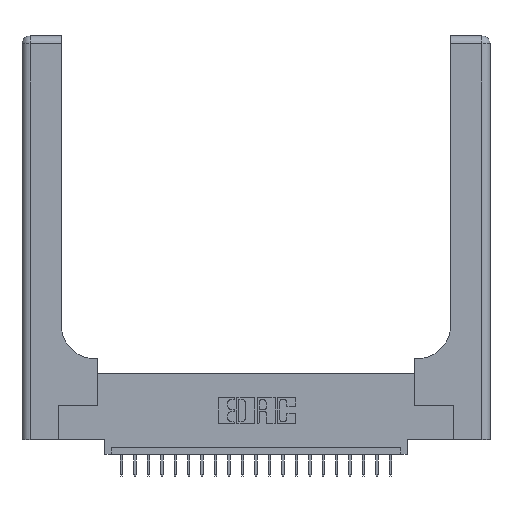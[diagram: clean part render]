
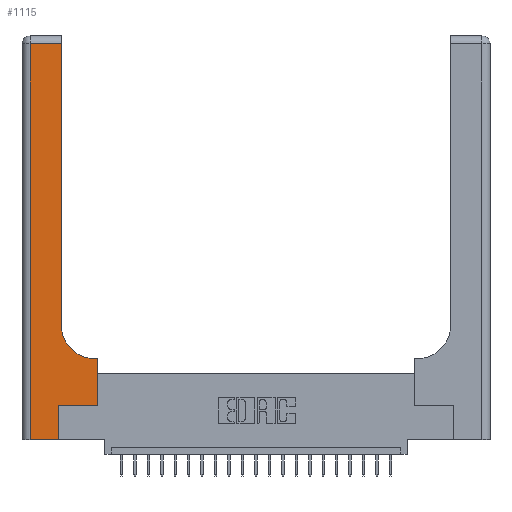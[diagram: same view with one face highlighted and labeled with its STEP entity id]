
A CAD part, top view. The second image highlights one B-rep face of the part: STEP entity #1115.
In plain terms, the highlighted planar face has unit normal (0, 0, 1).
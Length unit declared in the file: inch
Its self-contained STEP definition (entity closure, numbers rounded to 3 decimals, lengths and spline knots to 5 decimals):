
#96 = ORIENTED_EDGE ( 'NONE', *, *, #11299, .T. ) ;
#660 = VECTOR ( 'NONE', #7168, 39.37008 ) ;
#1115 = ADVANCED_FACE ( 'NONE', ( #14633 ), #4373, .F. ) ;
#1255 = VERTEX_POINT ( 'NONE', #6932 ) ;
#2038 = DIRECTION ( 'NONE',  ( 0., 1., 0. ) ) ;
#2277 = ORIENTED_EDGE ( 'NONE', *, *, #12733, .T. ) ;
#2320 = VECTOR ( 'NONE', #6712, 39.37008 ) ;
#2833 = DIRECTION ( 'NONE',  ( 1., 0., 0. ) ) ;
#3417 = ORIENTED_EDGE ( 'NONE', *, *, #20198, .T. ) ;
#3711 = DIRECTION ( 'NONE',  ( -1., 0., 0. ) ) ;
#3892 = ORIENTED_EDGE ( 'NONE', *, *, #22491, .T. ) ;
#4273 = EDGE_CURVE ( 'NONE', #1255, #19383, #12418, .T. ) ;
#4373 = PLANE ( 'NONE',  #24038 ) ;
#5080 = VECTOR ( 'NONE', #5881, 39.37008 ) ;
#5132 = EDGE_LOOP ( 'NONE', ( #2277, #96, #16296, #3892, #3417, #22652, #8991, #7483, #16198 ) ) ;
#5324 = LINE ( 'NONE', #10948, #6477 ) ;
#5587 = CARTESIAN_POINT ( 'NONE',  ( 0.2915, 0.85, 0.37 ) ) ;
#5657 = LINE ( 'NONE', #8108, #19506 ) ;
#5779 = AXIS2_PLACEMENT_3D ( 'NONE', #7704, #14783, #20620 ) ;
#5881 = DIRECTION ( 'NONE',  ( -1., 0., 0. ) ) ;
#6238 = CARTESIAN_POINT ( 'NONE',  ( 0., 3., 0.37 ) ) ;
#6273 = LINE ( 'NONE', #6801, #11749 ) ;
#6477 = VECTOR ( 'NONE', #2038, 39.37008 ) ;
#6712 = DIRECTION ( 'NONE',  ( 0., 1., 0. ) ) ;
#6801 = CARTESIAN_POINT ( 'NONE',  ( 0.269, 0., 0.37 ) ) ;
#6928 = CARTESIAN_POINT ( 'NONE',  ( 0.06, 2.94, 0.37 ) ) ;
#6932 = CARTESIAN_POINT ( 'NONE',  ( 0.5585, 0.25, 0.37 ) ) ;
#7168 = DIRECTION ( 'NONE',  ( 0., -1., 0. ) ) ;
#7483 = ORIENTED_EDGE ( 'NONE', *, *, #13497, .T. ) ;
#7704 = CARTESIAN_POINT ( 'NONE',  ( 0.5415, 0.85, 0.37 ) ) ;
#8108 = CARTESIAN_POINT ( 'NONE',  ( 0.269, 0.25, 0.37 ) ) ;
#8991 = ORIENTED_EDGE ( 'NONE', *, *, #4273, .T. ) ;
#10378 = VECTOR ( 'NONE', #14748, 39.37008 ) ;
#10526 = VERTEX_POINT ( 'NONE', #23783 ) ;
#10531 = VERTEX_POINT ( 'NONE', #14537 ) ;
#10604 = VERTEX_POINT ( 'NONE', #5587 ) ;
#10948 = CARTESIAN_POINT ( 'NONE',  ( 0.2915, 3., 0.37 ) ) ;
#11299 = EDGE_CURVE ( 'NONE', #10531, #23499, #14876, .T. ) ;
#11749 = VECTOR ( 'NONE', #21236, 39.37008 ) ;
#11845 = EDGE_CURVE ( 'NONE', #16604, #1255, #5657, .T. ) ;
#12418 = LINE ( 'NONE', #15806, #2320 ) ;
#12733 = EDGE_CURVE ( 'NONE', #10604, #10531, #5324, .T. ) ;
#12769 = VECTOR ( 'NONE', #3711, 39.37008 ) ;
#13497 = EDGE_CURVE ( 'NONE', #19383, #17892, #17670, .T. ) ;
#13524 = CARTESIAN_POINT ( 'NONE',  ( 0., 2.94, 0.37 ) ) ;
#13727 = DIRECTION ( 'NONE',  ( -1., 0., 0. ) ) ;
#13893 = EDGE_CURVE ( 'NONE', #17892, #10604, #22330, .T. ) ;
#14537 = CARTESIAN_POINT ( 'NONE',  ( 0.2915, 2.94, 0.37 ) ) ;
#14633 = FACE_OUTER_BOUND ( 'NONE', #5132, .T. ) ;
#14748 = DIRECTION ( 'NONE',  ( 1., 0., 0. ) ) ;
#14783 = DIRECTION ( 'NONE',  ( 0., 0., -1. ) ) ;
#14806 = CARTESIAN_POINT ( 'NONE',  ( 0.5585, 0.6, 0.37 ) ) ;
#14876 = LINE ( 'NONE', #13524, #5080 ) ;
#15123 = CARTESIAN_POINT ( 'NONE',  ( 0.269, 0.25, 0.37 ) ) ;
#15615 = EDGE_CURVE ( 'NONE', #23499, #16843, #17150, .T. ) ;
#15806 = CARTESIAN_POINT ( 'NONE',  ( 0.5585, 0.25, 0.37 ) ) ;
#16198 = ORIENTED_EDGE ( 'NONE', *, *, #13893, .T. ) ;
#16296 = ORIENTED_EDGE ( 'NONE', *, *, #15615, .T. ) ;
#16604 = VERTEX_POINT ( 'NONE', #15123 ) ;
#16655 = CARTESIAN_POINT ( 'NONE',  ( 0.06, 3., 0.37 ) ) ;
#16843 = VERTEX_POINT ( 'NONE', #21489 ) ;
#17150 = LINE ( 'NONE', #16655, #660 ) ;
#17456 = CARTESIAN_POINT ( 'NONE',  ( 0.5415, 0.6, 0.37 ) ) ;
#17670 = LINE ( 'NONE', #22539, #12769 ) ;
#17892 = VERTEX_POINT ( 'NONE', #17456 ) ;
#19132 = DIRECTION ( 'NONE',  ( 0., 0., -1. ) ) ;
#19383 = VERTEX_POINT ( 'NONE', #14806 ) ;
#19506 = VECTOR ( 'NONE', #2833, 39.37008 ) ;
#20198 = EDGE_CURVE ( 'NONE', #10526, #16604, #6273, .T. ) ;
#20620 = DIRECTION ( 'NONE',  ( 1., 0., 0. ) ) ;
#21236 = DIRECTION ( 'NONE',  ( 0., 1., 0. ) ) ;
#21489 = CARTESIAN_POINT ( 'NONE',  ( 0.06, 0., 0.37 ) ) ;
#22330 = CIRCLE ( 'NONE', #5779, 0.25 ) ;
#22491 = EDGE_CURVE ( 'NONE', #16843, #10526, #24022, .T. ) ;
#22539 = CARTESIAN_POINT ( 'NONE',  ( 0.2915, 0.6, 0.37 ) ) ;
#22652 = ORIENTED_EDGE ( 'NONE', *, *, #11845, .T. ) ;
#23499 = VERTEX_POINT ( 'NONE', #6928 ) ;
#23783 = CARTESIAN_POINT ( 'NONE',  ( 0.269, 0., 0.37 ) ) ;
#24022 = LINE ( 'NONE', #24026, #10378 ) ;
#24026 = CARTESIAN_POINT ( 'NONE',  ( 0., 0., 0.37 ) ) ;
#24038 = AXIS2_PLACEMENT_3D ( 'NONE', #6238, #19132, #13727 ) ;
